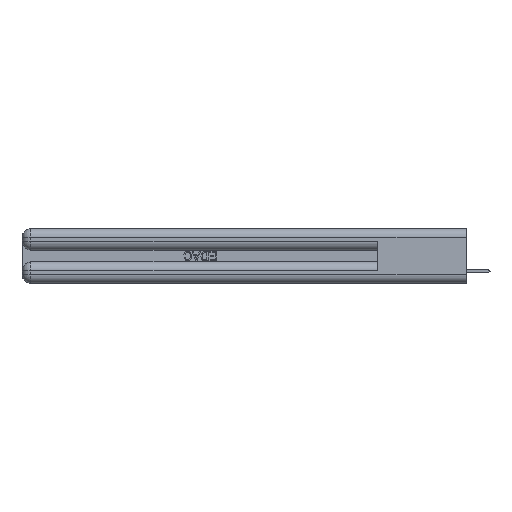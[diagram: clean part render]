
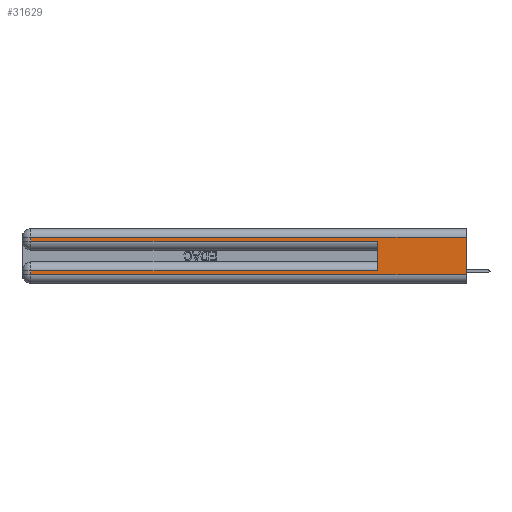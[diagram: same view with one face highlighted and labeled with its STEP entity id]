
A CAD part, left-side view. The second image highlights one B-rep face of the part: STEP entity #31629.
In plain terms, the highlighted planar face has unit normal (-1, 0, 0).
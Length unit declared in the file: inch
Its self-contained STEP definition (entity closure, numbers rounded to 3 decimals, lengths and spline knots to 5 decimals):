
#254 = CARTESIAN_POINT ( 'NONE',  ( 0., 0., 0.06 ) ) ;
#516 = EDGE_CURVE ( 'NONE', #5697, #1733, #39286, .T. ) ;
#893 = LINE ( 'NONE', #31699, #16248 ) ;
#1733 = VERTEX_POINT ( 'NONE', #2545 ) ;
#2037 = DIRECTION ( 'NONE',  ( 0., -1., 0. ) ) ;
#2269 = DIRECTION ( 'NONE',  ( 0., 0., -1. ) ) ;
#2318 = LINE ( 'NONE', #16272, #23019 ) ;
#2545 = CARTESIAN_POINT ( 'NONE',  ( 0., 2.94, 0.06 ) ) ;
#4904 = DIRECTION ( 'NONE',  ( 0., 1., 0. ) ) ;
#5697 = VERTEX_POINT ( 'NONE', #35683 ) ;
#6103 = ORIENTED_EDGE ( 'NONE', *, *, #35060, .T. ) ;
#6506 = FACE_OUTER_BOUND ( 'NONE', #25784, .T. ) ;
#6745 = PLANE ( 'NONE',  #32481 ) ;
#7187 = EDGE_CURVE ( 'NONE', #12610, #31097, #14433, .T. ) ;
#7299 = VECTOR ( 'NONE', #2269, 39.37008 ) ;
#8745 = VECTOR ( 'NONE', #20473, 39.37008 ) ;
#8768 = VECTOR ( 'NONE', #43800, 39.37008 ) ;
#9252 = CARTESIAN_POINT ( 'NONE',  ( 0., 0.6, 0.145 ) ) ;
#9601 = VERTEX_POINT ( 'NONE', #254 ) ;
#9721 = EDGE_CURVE ( 'NONE', #12875, #5697, #52141, .T. ) ;
#11559 = ORIENTED_EDGE ( 'NONE', *, *, #21278, .T. ) ;
#12610 = VERTEX_POINT ( 'NONE', #29409 ) ;
#12875 = VERTEX_POINT ( 'NONE', #48082 ) ;
#13242 = LINE ( 'NONE', #9252, #54700 ) ;
#14433 = LINE ( 'NONE', #52118, #29806 ) ;
#14480 = ORIENTED_EDGE ( 'NONE', *, *, #516, .T. ) ;
#16165 = CARTESIAN_POINT ( 'NONE',  ( 0., 0., 0.37 ) ) ;
#16248 = VECTOR ( 'NONE', #2037, 39.37008 ) ;
#16272 = CARTESIAN_POINT ( 'NONE',  ( 0., 0., 0.285 ) ) ;
#18605 = CARTESIAN_POINT ( 'NONE',  ( 0., 2.94, 0.285 ) ) ;
#19230 = CARTESIAN_POINT ( 'NONE',  ( 0., 2.94, 0.37 ) ) ;
#19390 = ORIENTED_EDGE ( 'NONE', *, *, #21608, .F. ) ;
#20408 = CARTESIAN_POINT ( 'NONE',  ( 0., 0.6, 0.285 ) ) ;
#20473 = DIRECTION ( 'NONE',  ( 0., 0., -1. ) ) ;
#20553 = DIRECTION ( 'NONE',  ( 0., 0., -1. ) ) ;
#21278 = EDGE_CURVE ( 'NONE', #1733, #9601, #893, .T. ) ;
#21608 = EDGE_CURVE ( 'NONE', #12610, #9601, #24693, .T. ) ;
#21873 = VECTOR ( 'NONE', #20553, 39.37008 ) ;
#22361 = ORIENTED_EDGE ( 'NONE', *, *, #7187, .T. ) ;
#23019 = VECTOR ( 'NONE', #25230, 39.37008 ) ;
#23284 = VERTEX_POINT ( 'NONE', #20408 ) ;
#23289 = DIRECTION ( 'NONE',  ( 1., 0., 0. ) ) ;
#23485 = ORIENTED_EDGE ( 'NONE', *, *, #51958, .F. ) ;
#24693 = LINE ( 'NONE', #16165, #8745 ) ;
#25230 = DIRECTION ( 'NONE',  ( 0., -1., 0. ) ) ;
#25784 = EDGE_LOOP ( 'NONE', ( #19390, #22361, #26039, #6103, #23485, #36958, #14480, #11559 ) ) ;
#26039 = ORIENTED_EDGE ( 'NONE', *, *, #39238, .T. ) ;
#29409 = CARTESIAN_POINT ( 'NONE',  ( 0., 0., 0.31 ) ) ;
#29806 = VECTOR ( 'NONE', #4904, 39.37008 ) ;
#31097 = VERTEX_POINT ( 'NONE', #36507 ) ;
#31629 = ADVANCED_FACE ( 'NONE', ( #6506 ), #6745, .F. ) ;
#31699 = CARTESIAN_POINT ( 'NONE',  ( 0., 0., 0.06 ) ) ;
#32256 = CARTESIAN_POINT ( 'NONE',  ( 0., 0., 0.37 ) ) ;
#32481 = AXIS2_PLACEMENT_3D ( 'NONE', #32256, #23289, #53589 ) ;
#33442 = CARTESIAN_POINT ( 'NONE',  ( 0., 2.94, 0.37 ) ) ;
#35060 = EDGE_CURVE ( 'NONE', #43797, #23284, #2318, .T. ) ;
#35203 = CARTESIAN_POINT ( 'NONE',  ( 0., 0., 0.085 ) ) ;
#35683 = CARTESIAN_POINT ( 'NONE',  ( 0., 2.94, 0.085 ) ) ;
#36507 = CARTESIAN_POINT ( 'NONE',  ( 0., 2.94, 0.31 ) ) ;
#36958 = ORIENTED_EDGE ( 'NONE', *, *, #9721, .T. ) ;
#39238 = EDGE_CURVE ( 'NONE', #31097, #43797, #53356, .T. ) ;
#39286 = LINE ( 'NONE', #33442, #21873 ) ;
#43238 = DIRECTION ( 'NONE',  ( 0., 0., 1. ) ) ;
#43797 = VERTEX_POINT ( 'NONE', #18605 ) ;
#43800 = DIRECTION ( 'NONE',  ( 0., 1., 0. ) ) ;
#48082 = CARTESIAN_POINT ( 'NONE',  ( 0., 0.6, 0.085 ) ) ;
#51958 = EDGE_CURVE ( 'NONE', #12875, #23284, #13242, .T. ) ;
#52118 = CARTESIAN_POINT ( 'NONE',  ( 0., 0., 0.31 ) ) ;
#52141 = LINE ( 'NONE', #35203, #8768 ) ;
#53356 = LINE ( 'NONE', #19230, #7299 ) ;
#53589 = DIRECTION ( 'NONE',  ( 0., 0., -1. ) ) ;
#54700 = VECTOR ( 'NONE', #43238, 39.37008 ) ;
